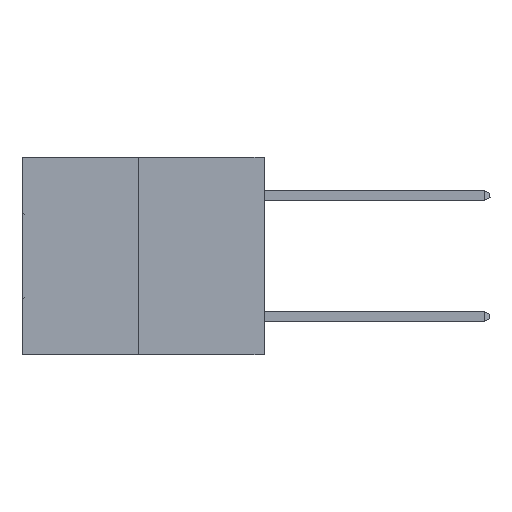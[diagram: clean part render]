
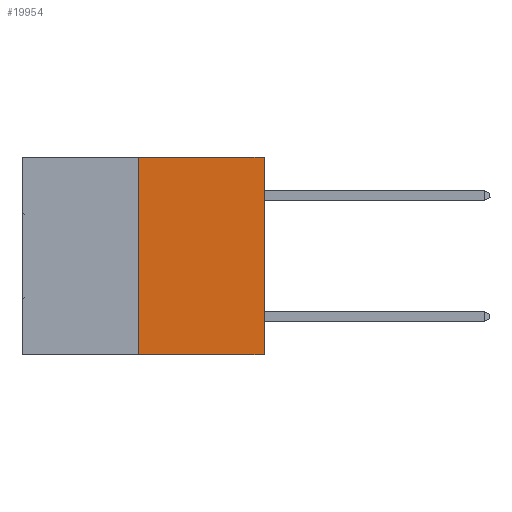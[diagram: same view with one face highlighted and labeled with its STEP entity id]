
A CAD part, left-side view. The second image highlights one B-rep face of the part: STEP entity #19954.
In plain terms, the highlighted planar face has unit normal (-1, 0, 0).
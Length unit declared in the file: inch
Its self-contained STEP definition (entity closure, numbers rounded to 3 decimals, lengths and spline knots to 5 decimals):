
#661 = EDGE_LOOP ( 'NONE', ( #3085, #33241, #10528, #25234 ) ) ;
#1150 = DIRECTION ( 'NONE',  ( 0., 0., 1. ) ) ;
#2024 = EDGE_CURVE ( 'NONE', #14335, #27220, #24527, .T. ) ;
#3066 = CARTESIAN_POINT ( 'NONE',  ( 0., 0., 0. ) ) ;
#3085 = ORIENTED_EDGE ( 'NONE', *, *, #2024, .F. ) ;
#3997 = VERTEX_POINT ( 'NONE', #32112 ) ;
#5341 = AXIS2_PLACEMENT_3D ( 'NONE', #9355, #17401, #17525 ) ;
#8747 = CARTESIAN_POINT ( 'NONE',  ( 0., 0.6, -0.49 ) ) ;
#9355 = CARTESIAN_POINT ( 'NONE',  ( 0., 0.6, 0. ) ) ;
#10401 = VECTOR ( 'NONE', #17128, 39.37008 ) ;
#10528 = ORIENTED_EDGE ( 'NONE', *, *, #26947, .T. ) ;
#11233 = EDGE_CURVE ( 'NONE', #14335, #34668, #32256, .T. ) ;
#12323 = FACE_OUTER_BOUND ( 'NONE', #661, .T. ) ;
#12733 = CARTESIAN_POINT ( 'NONE',  ( 0., 0.6, 0. ) ) ;
#14335 = VERTEX_POINT ( 'NONE', #14491 ) ;
#14491 = CARTESIAN_POINT ( 'NONE',  ( 0., 0.312, -0.49 ) ) ;
#14919 = CARTESIAN_POINT ( 'NONE',  ( 0., 0.312, 0. ) ) ;
#15763 = CARTESIAN_POINT ( 'NONE',  ( 0., 0.312, -0.49 ) ) ;
#17128 = DIRECTION ( 'NONE',  ( 0., -1., 0. ) ) ;
#17401 = DIRECTION ( 'NONE',  ( 1., 0., 0. ) ) ;
#17525 = DIRECTION ( 'NONE',  ( 0., 0., -1. ) ) ;
#17591 = LINE ( 'NONE', #3066, #31573 ) ;
#19329 = EDGE_CURVE ( 'NONE', #27220, #3997, #29789, .T. ) ;
#19954 = ADVANCED_FACE ( 'NONE', ( #12323 ), #31830, .F. ) ;
#22782 = VECTOR ( 'NONE', #29806, 39.37008 ) ;
#24527 = LINE ( 'NONE', #15763, #22782 ) ;
#25234 = ORIENTED_EDGE ( 'NONE', *, *, #19329, .F. ) ;
#26947 = EDGE_CURVE ( 'NONE', #34668, #3997, #17591, .T. ) ;
#27220 = VERTEX_POINT ( 'NONE', #14919 ) ;
#28493 = VECTOR ( 'NONE', #30044, 39.37008 ) ;
#29180 = CARTESIAN_POINT ( 'NONE',  ( 0., 0., -0.49 ) ) ;
#29789 = LINE ( 'NONE', #12733, #28493 ) ;
#29806 = DIRECTION ( 'NONE',  ( 0., 0., 1. ) ) ;
#30044 = DIRECTION ( 'NONE',  ( 0., -1., 0. ) ) ;
#31573 = VECTOR ( 'NONE', #1150, 39.37008 ) ;
#31830 = PLANE ( 'NONE',  #5341 ) ;
#32112 = CARTESIAN_POINT ( 'NONE',  ( 0., 0., 0. ) ) ;
#32256 = LINE ( 'NONE', #8747, #10401 ) ;
#33241 = ORIENTED_EDGE ( 'NONE', *, *, #11233, .T. ) ;
#34668 = VERTEX_POINT ( 'NONE', #29180 ) ;
